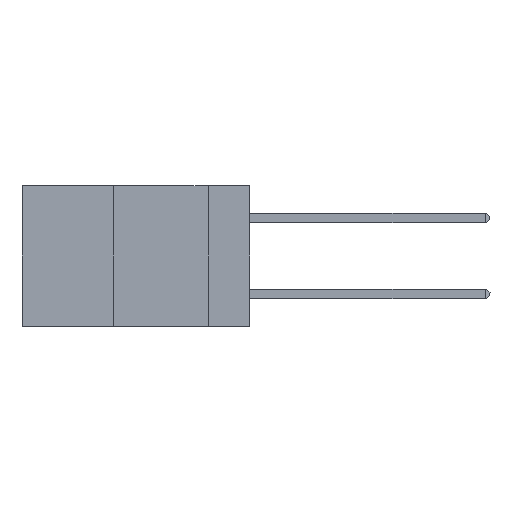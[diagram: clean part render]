
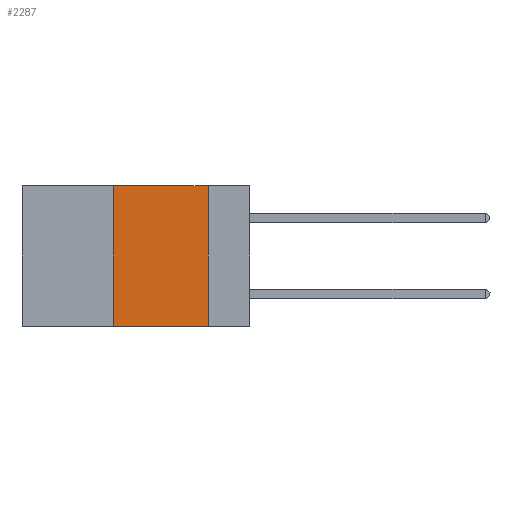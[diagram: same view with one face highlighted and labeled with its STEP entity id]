
A CAD part, left-side view. The second image highlights one B-rep face of the part: STEP entity #2287.
In plain terms, the highlighted planar face has unit normal (-1, 0, 0).
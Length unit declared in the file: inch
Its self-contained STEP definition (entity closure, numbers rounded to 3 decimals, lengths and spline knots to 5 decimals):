
#51 = VERTEX_POINT ( 'NONE', #3850 ) ;
#808 = ORIENTED_EDGE ( 'NONE', *, *, #10501, .F. ) ;
#1097 = CARTESIAN_POINT ( 'NONE',  ( 0., 0.11, 0. ) ) ;
#1384 = CARTESIAN_POINT ( 'NONE',  ( 0., 0.36, -0.37 ) ) ;
#1626 = LINE ( 'NONE', #4403, #9556 ) ;
#2287 = ADVANCED_FACE ( 'NONE', ( #3777 ), #11582, .F. ) ;
#2305 = CARTESIAN_POINT ( 'NONE',  ( 0., 0.6, 0. ) ) ;
#3211 = EDGE_LOOP ( 'NONE', ( #6238, #11545, #808, #7440 ) ) ;
#3777 = FACE_OUTER_BOUND ( 'NONE', #3211, .T. ) ;
#3850 = CARTESIAN_POINT ( 'NONE',  ( 0., 0.11, -0.37 ) ) ;
#4258 = LINE ( 'NONE', #5020, #5813 ) ;
#4403 = CARTESIAN_POINT ( 'NONE',  ( 0., 0.6, -0.37 ) ) ;
#5006 = DIRECTION ( 'NONE',  ( 0., 0., 1. ) ) ;
#5020 = CARTESIAN_POINT ( 'NONE',  ( 0., 0.6, 0. ) ) ;
#5130 = VERTEX_POINT ( 'NONE', #8052 ) ;
#5744 = VERTEX_POINT ( 'NONE', #9146 ) ;
#5813 = VECTOR ( 'NONE', #8294, 39.37008 ) ;
#6238 = ORIENTED_EDGE ( 'NONE', *, *, #12301, .F. ) ;
#6377 = LINE ( 'NONE', #12347, #8452 ) ;
#6431 = DIRECTION ( 'NONE',  ( 0., 0., -1. ) ) ;
#7440 = ORIENTED_EDGE ( 'NONE', *, *, #14012, .T. ) ;
#7779 = EDGE_CURVE ( 'NONE', #5744, #5130, #4258, .T. ) ;
#8052 = CARTESIAN_POINT ( 'NONE',  ( 0., 0.11, 0. ) ) ;
#8294 = DIRECTION ( 'NONE',  ( 0., -1., 0. ) ) ;
#8452 = VECTOR ( 'NONE', #5006, 39.37008 ) ;
#8578 = DIRECTION ( 'NONE',  ( 0., 0., -1. ) ) ;
#8852 = DIRECTION ( 'NONE',  ( 1., 0., 0. ) ) ;
#9146 = CARTESIAN_POINT ( 'NONE',  ( 0., 0.36, 0. ) ) ;
#9556 = VECTOR ( 'NONE', #13305, 39.37008 ) ;
#10501 = EDGE_CURVE ( 'NONE', #11844, #5744, #6377, .T. ) ;
#10817 = AXIS2_PLACEMENT_3D ( 'NONE', #2305, #8852, #8578 ) ;
#11463 = VECTOR ( 'NONE', #6431, 39.37008 ) ;
#11545 = ORIENTED_EDGE ( 'NONE', *, *, #7779, .F. ) ;
#11582 = PLANE ( 'NONE',  #10817 ) ;
#11844 = VERTEX_POINT ( 'NONE', #1384 ) ;
#12152 = LINE ( 'NONE', #1097, #11463 ) ;
#12301 = EDGE_CURVE ( 'NONE', #5130, #51, #12152, .T. ) ;
#12347 = CARTESIAN_POINT ( 'NONE',  ( 0., 0.36, 0. ) ) ;
#13305 = DIRECTION ( 'NONE',  ( 0., -1., 0. ) ) ;
#14012 = EDGE_CURVE ( 'NONE', #11844, #51, #1626, .T. ) ;
